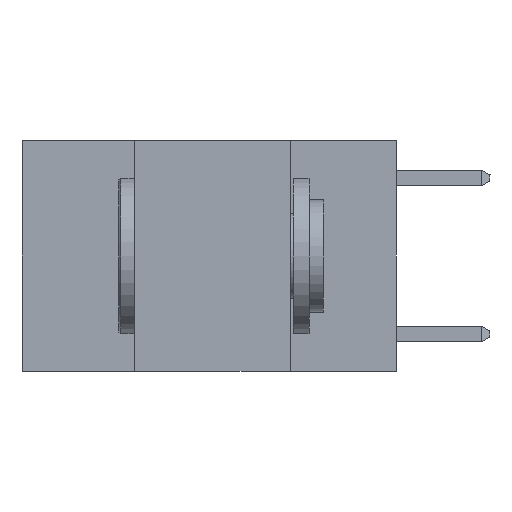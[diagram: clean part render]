
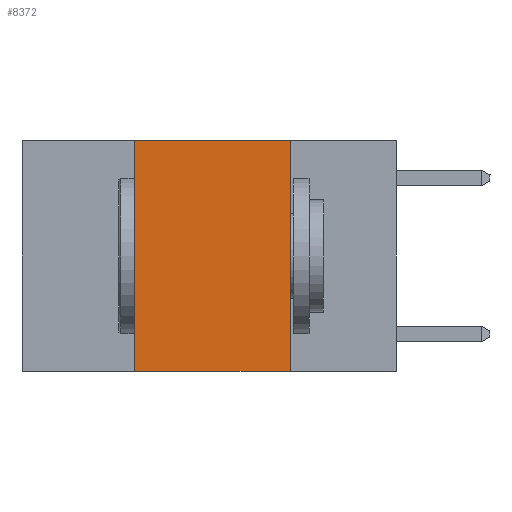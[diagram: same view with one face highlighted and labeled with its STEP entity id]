
A CAD part, left-side view. The second image highlights one B-rep face of the part: STEP entity #8372.
In plain terms, the highlighted planar face has unit normal (-1, 0, 0).
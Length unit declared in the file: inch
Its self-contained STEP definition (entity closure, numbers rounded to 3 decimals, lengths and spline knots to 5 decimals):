
#296 = LINE ( 'NONE', #12136, #12978 ) ;
#434 = CARTESIAN_POINT ( 'NONE',  ( 0., 0.42, 0. ) ) ;
#518 = CARTESIAN_POINT ( 'NONE',  ( 0., 0.6, 0. ) ) ;
#1391 = CARTESIAN_POINT ( 'NONE',  ( 0., 0.17, 0. ) ) ;
#1971 = VERTEX_POINT ( 'NONE', #434 ) ;
#2025 = LINE ( 'NONE', #15233, #8954 ) ;
#2210 = DIRECTION ( 'NONE',  ( 0., 0., -1. ) ) ;
#3463 = PLANE ( 'NONE',  #8729 ) ;
#3523 = DIRECTION ( 'NONE',  ( 0., 0., 1. ) ) ;
#3678 = VECTOR ( 'NONE', #2210, 39.37008 ) ;
#3852 = DIRECTION ( 'NONE',  ( 1., 0., 0. ) ) ;
#6255 = ORIENTED_EDGE ( 'NONE', *, *, #18034, .F. ) ;
#6578 = CARTESIAN_POINT ( 'NONE',  ( 0., 0.17, -0.37 ) ) ;
#7394 = VERTEX_POINT ( 'NONE', #6578 ) ;
#7535 = CARTESIAN_POINT ( 'NONE',  ( 0., 0.42, 0. ) ) ;
#7623 = CARTESIAN_POINT ( 'NONE',  ( 0., 0.42, -0.37 ) ) ;
#7691 = EDGE_CURVE ( 'NONE', #17248, #1971, #16532, .T. ) ;
#8372 = ADVANCED_FACE ( 'NONE', ( #11091 ), #3463, .F. ) ;
#8729 = AXIS2_PLACEMENT_3D ( 'NONE', #518, #3852, #18730 ) ;
#8954 = VECTOR ( 'NONE', #14162, 39.37008 ) ;
#9277 = EDGE_LOOP ( 'NONE', ( #6255, #16595, #15982, #11268 ) ) ;
#9660 = LINE ( 'NONE', #11016, #3678 ) ;
#11016 = CARTESIAN_POINT ( 'NONE',  ( 0., 0.17, 0. ) ) ;
#11091 = FACE_OUTER_BOUND ( 'NONE', #9277, .T. ) ;
#11268 = ORIENTED_EDGE ( 'NONE', *, *, #15379, .T. ) ;
#11626 = VERTEX_POINT ( 'NONE', #1391 ) ;
#12136 = CARTESIAN_POINT ( 'NONE',  ( 0., 0.6, -0.37 ) ) ;
#12978 = VECTOR ( 'NONE', #13509, 39.37008 ) ;
#13509 = DIRECTION ( 'NONE',  ( 0., -1., 0. ) ) ;
#14162 = DIRECTION ( 'NONE',  ( 0., -1., 0. ) ) ;
#14561 = VECTOR ( 'NONE', #3523, 39.37008 ) ;
#15233 = CARTESIAN_POINT ( 'NONE',  ( 0., 0.6, 0. ) ) ;
#15379 = EDGE_CURVE ( 'NONE', #17248, #7394, #296, .T. ) ;
#15982 = ORIENTED_EDGE ( 'NONE', *, *, #7691, .F. ) ;
#16099 = EDGE_CURVE ( 'NONE', #1971, #11626, #2025, .T. ) ;
#16532 = LINE ( 'NONE', #7535, #14561 ) ;
#16595 = ORIENTED_EDGE ( 'NONE', *, *, #16099, .F. ) ;
#17248 = VERTEX_POINT ( 'NONE', #7623 ) ;
#18034 = EDGE_CURVE ( 'NONE', #11626, #7394, #9660, .T. ) ;
#18730 = DIRECTION ( 'NONE',  ( 0., 0., -1. ) ) ;
